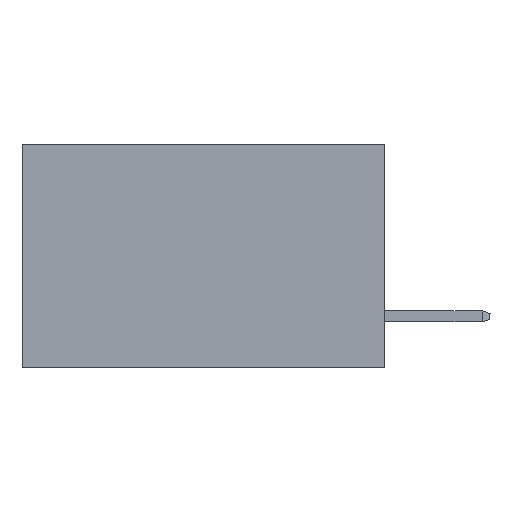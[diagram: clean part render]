
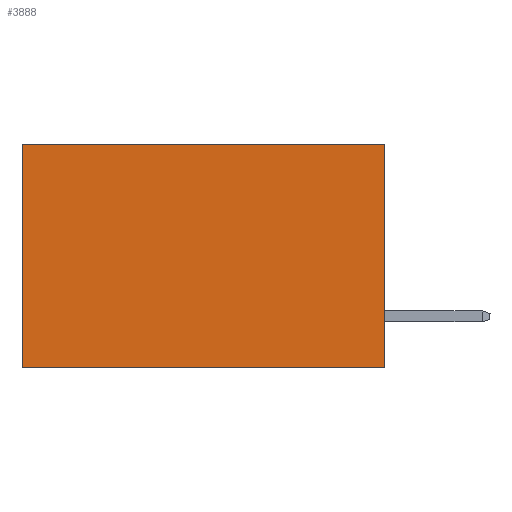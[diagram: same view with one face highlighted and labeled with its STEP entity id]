
A CAD part, left-side view. The second image highlights one B-rep face of the part: STEP entity #3888.
In plain terms, the highlighted planar face has unit normal (-1, 0, 0).
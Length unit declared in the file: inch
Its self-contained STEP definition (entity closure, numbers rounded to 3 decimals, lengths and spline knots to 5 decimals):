
#388 = ORIENTED_EDGE ( 'NONE', *, *, #7087, .T. ) ;
#898 = EDGE_CURVE ( 'NONE', #6635, #10517, #7791, .T. ) ;
#937 = VECTOR ( 'NONE', #7945, 39.37008 ) ;
#1469 = VERTEX_POINT ( 'NONE', #3269 ) ;
#1906 = VECTOR ( 'NONE', #7613, 39.37008 ) ;
#2018 = ORIENTED_EDGE ( 'NONE', *, *, #13019, .T. ) ;
#2740 = LINE ( 'NONE', #11168, #7398 ) ;
#3269 = CARTESIAN_POINT ( 'NONE',  ( 0.2615, 0.6, 0. ) ) ;
#3592 = DIRECTION ( 'NONE',  ( 0., 1., 0. ) ) ;
#3669 = CARTESIAN_POINT ( 'NONE',  ( 0.2615, 0., -0.37 ) ) ;
#3888 = ADVANCED_FACE ( 'NONE', ( #10519 ), #6100, .F. ) ;
#3978 = DIRECTION ( 'NONE',  ( 0., 0., -1. ) ) ;
#4115 = CARTESIAN_POINT ( 'NONE',  ( 0.2615, 0.6, -0.37 ) ) ;
#6100 = PLANE ( 'NONE',  #7857 ) ;
#6214 = ORIENTED_EDGE ( 'NONE', *, *, #12377, .F. ) ;
#6635 = VERTEX_POINT ( 'NONE', #10667 ) ;
#6707 = ORIENTED_EDGE ( 'NONE', *, *, #898, .F. ) ;
#7087 = EDGE_CURVE ( 'NONE', #1469, #13515, #13820, .T. ) ;
#7398 = VECTOR ( 'NONE', #3592, 39.37008 ) ;
#7406 = CARTESIAN_POINT ( 'NONE',  ( 0.2615, 0., -0.37 ) ) ;
#7547 = CARTESIAN_POINT ( 'NONE',  ( 0.2615, 0., -0.37 ) ) ;
#7613 = DIRECTION ( 'NONE',  ( 0., 0., -1. ) ) ;
#7791 = LINE ( 'NONE', #3669, #937 ) ;
#7857 = AXIS2_PLACEMENT_3D ( 'NONE', #10395, #12504, #3978 ) ;
#7945 = DIRECTION ( 'NONE',  ( 0., 0., -1. ) ) ;
#8088 = EDGE_LOOP ( 'NONE', ( #388, #6214, #6707, #2018 ) ) ;
#8616 = DIRECTION ( 'NONE',  ( 0., 1., 0. ) ) ;
#10395 = CARTESIAN_POINT ( 'NONE',  ( 0.2615, 0., -0.37 ) ) ;
#10517 = VERTEX_POINT ( 'NONE', #7547 ) ;
#10519 = FACE_OUTER_BOUND ( 'NONE', #8088, .T. ) ;
#10667 = CARTESIAN_POINT ( 'NONE',  ( 0.2615, 0., 0. ) ) ;
#10776 = LINE ( 'NONE', #7406, #13035 ) ;
#11168 = CARTESIAN_POINT ( 'NONE',  ( 0.2615, 0., 0. ) ) ;
#12377 = EDGE_CURVE ( 'NONE', #10517, #13515, #10776, .T. ) ;
#12491 = CARTESIAN_POINT ( 'NONE',  ( 0.2615, 0.6, -0.37 ) ) ;
#12504 = DIRECTION ( 'NONE',  ( 1., 0., 0. ) ) ;
#13019 = EDGE_CURVE ( 'NONE', #6635, #1469, #2740, .T. ) ;
#13035 = VECTOR ( 'NONE', #8616, 39.37008 ) ;
#13515 = VERTEX_POINT ( 'NONE', #12491 ) ;
#13820 = LINE ( 'NONE', #4115, #1906 ) ;
